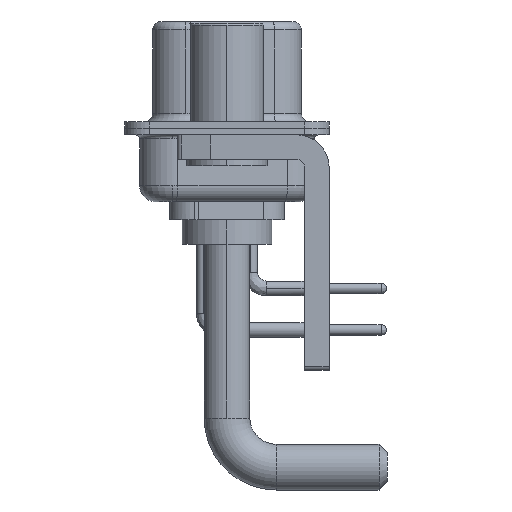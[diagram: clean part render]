
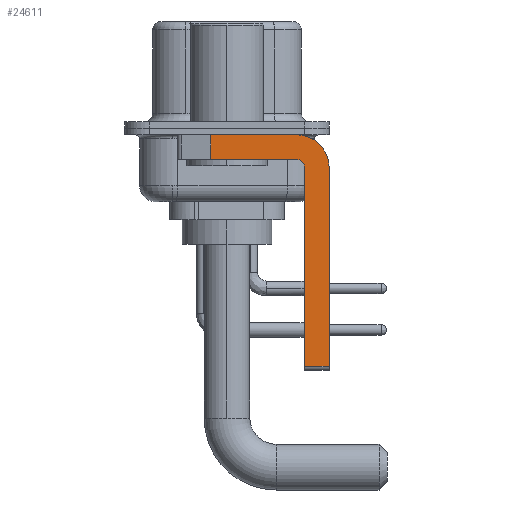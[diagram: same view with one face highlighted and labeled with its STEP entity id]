
A CAD part, left-side view. The second image highlights one B-rep face of the part: STEP entity #24611.
In plain terms, the highlighted planar face has unit normal (-1, 0, 0).
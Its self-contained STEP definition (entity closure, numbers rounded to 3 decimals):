
#458 = ORIENTED_EDGE ( 'NONE', *, *, #12052, .T. ) ;
#745 = CARTESIAN_POINT ( 'NONE',  ( -2.9, -4.25, -1.9 ) ) ;
#1006 = CIRCLE ( 'NONE', #6693, 0.5 ) ;
#1465 = VECTOR ( 'NONE', #7939, 1000. ) ;
#2679 = DIRECTION ( 'NONE',  ( 1., 0., 0. ) ) ;
#3318 = ORIENTED_EDGE ( 'NONE', *, *, #16382, .F. ) ;
#4350 = CARTESIAN_POINT ( 'NONE',  ( -2.9, -4.25, -2.4 ) ) ;
#4476 = CARTESIAN_POINT ( 'NONE',  ( -2.9, -4.25, -2.4 ) ) ;
#4641 = LINE ( 'NONE', #12965, #8920 ) ;
#5520 = CARTESIAN_POINT ( 'NONE',  ( -2.9, -4.25, -2.4 ) ) ;
#5656 = VECTOR ( 'NONE', #21723, 1000. ) ;
#6693 = AXIS2_PLACEMENT_3D ( 'NONE', #5520, #18076, #22192 ) ;
#6740 = CARTESIAN_POINT ( 'NONE',  ( -2.9, 0.978, -1.9 ) ) ;
#6762 = VERTEX_POINT ( 'NONE', #745 ) ;
#7238 = VERTEX_POINT ( 'NONE', #6740 ) ;
#7278 = VECTOR ( 'NONE', #8028, 1000. ) ;
#7296 = CARTESIAN_POINT ( 'NONE',  ( -2.9, -6.25, -2.4 ) ) ;
#7478 = AXIS2_PLACEMENT_3D ( 'NONE', #4476, #2679, #25216 ) ;
#7874 = LINE ( 'NONE', #14297, #8350 ) ;
#7939 = DIRECTION ( 'NONE',  ( 0., -1., 0. ) ) ;
#8028 = DIRECTION ( 'NONE',  ( 0., 0., 1. ) ) ;
#8350 = VECTOR ( 'NONE', #22632, 1000. ) ;
#8920 = VECTOR ( 'NONE', #17455, 1000. ) ;
#9647 = EDGE_CURVE ( 'NONE', #6762, #7238, #24395, .T. ) ;
#9733 = EDGE_CURVE ( 'NONE', #21611, #13220, #7874, .T. ) ;
#11019 = FACE_OUTER_BOUND ( 'NONE', #15222, .T. ) ;
#11475 = CARTESIAN_POINT ( 'NONE',  ( -2.9, -4.75, -2.4 ) ) ;
#11699 = DIRECTION ( 'NONE',  ( 0., 1., 0. ) ) ;
#11936 = ORIENTED_EDGE ( 'NONE', *, *, #20841, .F. ) ;
#12052 = EDGE_CURVE ( 'NONE', #18948, #13220, #16280, .T. ) ;
#12823 = DIRECTION ( 'NONE',  ( 1., 0., 0. ) ) ;
#12858 = EDGE_CURVE ( 'NONE', #14527, #7238, #4641, .T. ) ;
#12965 = CARTESIAN_POINT ( 'NONE',  ( -2.9, 0.978, -1.9 ) ) ;
#13220 = VERTEX_POINT ( 'NONE', #21286 ) ;
#14297 = CARTESIAN_POINT ( 'NONE',  ( -2.9, -6.25, -2.4 ) ) ;
#14527 = VERTEX_POINT ( 'NONE', #20510 ) ;
#15222 = EDGE_LOOP ( 'NONE', ( #11936, #26100, #21407, #21965, #16849, #458, #17341, #3318 ) ) ;
#16164 = EDGE_CURVE ( 'NONE', #18948, #17958, #26880, .T. ) ;
#16280 = LINE ( 'NONE', #26918, #1465 ) ;
#16382 = EDGE_CURVE ( 'NONE', #25304, #21611, #20794, .T. ) ;
#16849 = ORIENTED_EDGE ( 'NONE', *, *, #16164, .F. ) ;
#17208 = LINE ( 'NONE', #19661, #5656 ) ;
#17341 = ORIENTED_EDGE ( 'NONE', *, *, #9733, .F. ) ;
#17455 = DIRECTION ( 'NONE',  ( 0., 0., -1. ) ) ;
#17958 = VERTEX_POINT ( 'NONE', #11475 ) ;
#18076 = DIRECTION ( 'NONE',  ( -1., 0., 0. ) ) ;
#18590 = AXIS2_PLACEMENT_3D ( 'NONE', #4350, #12823, #21435 ) ;
#18948 = VERTEX_POINT ( 'NONE', #25008 ) ;
#19493 = PLANE ( 'NONE',  #7478 ) ;
#19661 = CARTESIAN_POINT ( 'NONE',  ( -2.9, 3., -0.4 ) ) ;
#20510 = CARTESIAN_POINT ( 'NONE',  ( -2.9, 0.978, -0.4 ) ) ;
#20794 = CIRCLE ( 'NONE', #18590, 2. ) ;
#20841 = EDGE_CURVE ( 'NONE', #14527, #25304, #17208, .T. ) ;
#21286 = CARTESIAN_POINT ( 'NONE',  ( -2.9, -6.25, -14.55 ) ) ;
#21407 = ORIENTED_EDGE ( 'NONE', *, *, #9647, .F. ) ;
#21435 = DIRECTION ( 'NONE',  ( 0., 0., -1. ) ) ;
#21474 = VECTOR ( 'NONE', #11699, 1000. ) ;
#21611 = VERTEX_POINT ( 'NONE', #7296 ) ;
#21723 = DIRECTION ( 'NONE',  ( 0., -1., 0. ) ) ;
#21965 = ORIENTED_EDGE ( 'NONE', *, *, #26110, .F. ) ;
#22103 = CARTESIAN_POINT ( 'NONE',  ( -2.9, -4.25, -1.9 ) ) ;
#22192 = DIRECTION ( 'NONE',  ( 0., 0., 1. ) ) ;
#22632 = DIRECTION ( 'NONE',  ( 0., 0., -1. ) ) ;
#24146 = CARTESIAN_POINT ( 'NONE',  ( -2.9, -4.25, -0.4 ) ) ;
#24395 = LINE ( 'NONE', #22103, #21474 ) ;
#24611 = ADVANCED_FACE ( 'NONE', ( #11019 ), #19493, .F. ) ;
#25008 = CARTESIAN_POINT ( 'NONE',  ( -2.9, -4.75, -14.55 ) ) ;
#25216 = DIRECTION ( 'NONE',  ( 0., 0., -1. ) ) ;
#25304 = VERTEX_POINT ( 'NONE', #24146 ) ;
#26100 = ORIENTED_EDGE ( 'NONE', *, *, #12858, .T. ) ;
#26110 = EDGE_CURVE ( 'NONE', #17958, #6762, #1006, .T. ) ;
#26472 = CARTESIAN_POINT ( 'NONE',  ( -2.9, -4.75, -14.8 ) ) ;
#26880 = LINE ( 'NONE', #26472, #7278 ) ;
#26918 = CARTESIAN_POINT ( 'NONE',  ( -2.9, -4.25, -14.55 ) ) ;
